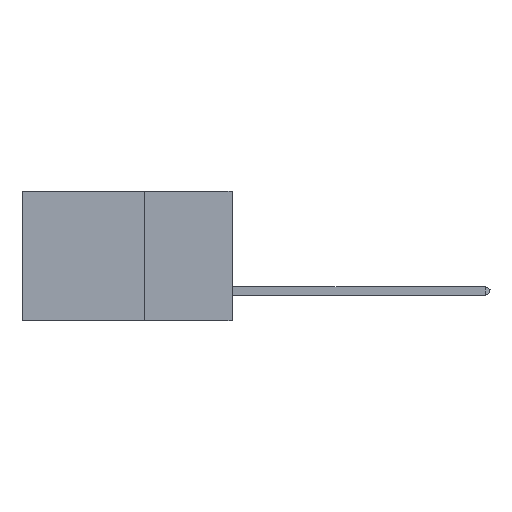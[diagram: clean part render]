
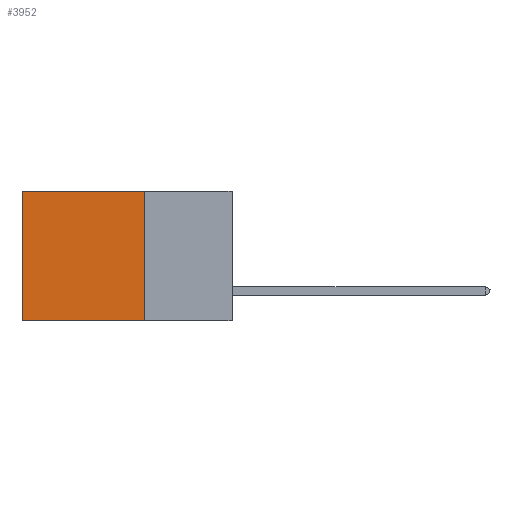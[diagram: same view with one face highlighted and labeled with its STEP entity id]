
A CAD part, left-side view. The second image highlights one B-rep face of the part: STEP entity #3952.
In plain terms, the highlighted planar face has unit normal (-1, 0, 0).
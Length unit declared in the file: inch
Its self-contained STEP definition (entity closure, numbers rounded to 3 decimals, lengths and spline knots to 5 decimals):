
#848 = DIRECTION ( 'NONE',  ( 0., 0., -1. ) ) ;
#1556 = CARTESIAN_POINT ( 'NONE',  ( 0.2875, 0.6, 0. ) ) ;
#3617 = DIRECTION ( 'NONE',  ( 0., 0., -1. ) ) ;
#3952 = ADVANCED_FACE ( 'NONE', ( #8843 ), #13097, .F. ) ;
#5578 = VECTOR ( 'NONE', #7825, 39.37008 ) ;
#7190 = EDGE_CURVE ( 'NONE', #17462, #25350, #24763, .T. ) ;
#7825 = DIRECTION ( 'NONE',  ( 0., 1., 0. ) ) ;
#8843 = FACE_OUTER_BOUND ( 'NONE', #25879, .T. ) ;
#9294 = ORIENTED_EDGE ( 'NONE', *, *, #25600, .F. ) ;
#10724 = EDGE_CURVE ( 'NONE', #18282, #16815, #36749, .T. ) ;
#12903 = ORIENTED_EDGE ( 'NONE', *, *, #31860, .T. ) ;
#13097 = PLANE ( 'NONE',  #36508 ) ;
#13634 = CARTESIAN_POINT ( 'NONE',  ( 0.2875, 0.25, 0. ) ) ;
#15853 = CARTESIAN_POINT ( 'NONE',  ( 0.2875, 0.25, -0.37 ) ) ;
#16815 = VERTEX_POINT ( 'NONE', #1556 ) ;
#17462 = VERTEX_POINT ( 'NONE', #15853 ) ;
#18282 = VERTEX_POINT ( 'NONE', #27457 ) ;
#18297 = CARTESIAN_POINT ( 'NONE',  ( 0.2875, 0.25, 0. ) ) ;
#19821 = VECTOR ( 'NONE', #21981, 39.37008 ) ;
#20483 = DIRECTION ( 'NONE',  ( 1., 0., 0. ) ) ;
#20749 = CARTESIAN_POINT ( 'NONE',  ( 0.2875, 0.6, 0. ) ) ;
#21629 = LINE ( 'NONE', #13634, #19821 ) ;
#21981 = DIRECTION ( 'NONE',  ( 0., 0., -1. ) ) ;
#23551 = ORIENTED_EDGE ( 'NONE', *, *, #7190, .F. ) ;
#23841 = CARTESIAN_POINT ( 'NONE',  ( 0.2875, 0.25, 0. ) ) ;
#24763 = LINE ( 'NONE', #27384, #5578 ) ;
#25350 = VERTEX_POINT ( 'NONE', #32461 ) ;
#25600 = EDGE_CURVE ( 'NONE', #18282, #17462, #21629, .T. ) ;
#25879 = EDGE_LOOP ( 'NONE', ( #12903, #23551, #9294, #36343 ) ) ;
#27384 = CARTESIAN_POINT ( 'NONE',  ( 0.2875, 0.25, -0.37 ) ) ;
#27457 = CARTESIAN_POINT ( 'NONE',  ( 0.2875, 0.25, 0. ) ) ;
#28470 = LINE ( 'NONE', #20749, #34640 ) ;
#29066 = VECTOR ( 'NONE', #35404, 39.37008 ) ;
#31860 = EDGE_CURVE ( 'NONE', #16815, #25350, #28470, .T. ) ;
#32461 = CARTESIAN_POINT ( 'NONE',  ( 0.2875, 0.6, -0.37 ) ) ;
#34640 = VECTOR ( 'NONE', #3617, 39.37008 ) ;
#35404 = DIRECTION ( 'NONE',  ( 0., 1., 0. ) ) ;
#36343 = ORIENTED_EDGE ( 'NONE', *, *, #10724, .T. ) ;
#36508 = AXIS2_PLACEMENT_3D ( 'NONE', #18297, #20483, #848 ) ;
#36749 = LINE ( 'NONE', #23841, #29066 ) ;
